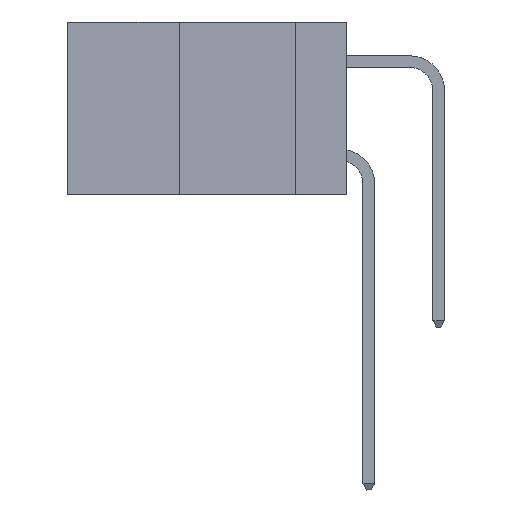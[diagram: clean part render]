
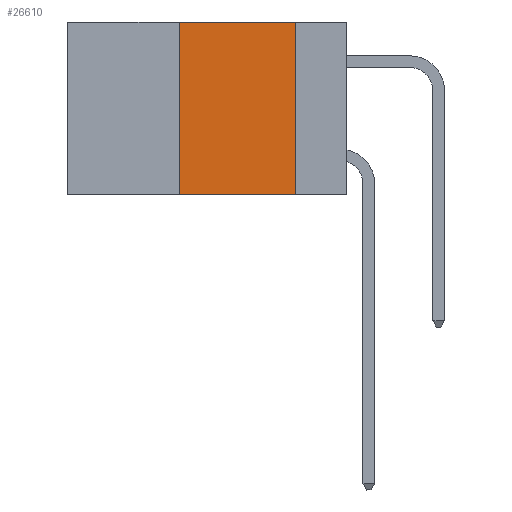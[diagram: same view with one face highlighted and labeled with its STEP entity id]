
A CAD part, left-side view. The second image highlights one B-rep face of the part: STEP entity #26610.
In plain terms, the highlighted planar face has unit normal (-1, 0, 0).
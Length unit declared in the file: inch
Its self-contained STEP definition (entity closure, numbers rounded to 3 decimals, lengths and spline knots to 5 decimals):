
#167 = CARTESIAN_POINT ( 'NONE',  ( 0., 0.6, 0. ) ) ;
#699 = ORIENTED_EDGE ( 'NONE', *, *, #12924, .T. ) ;
#1971 = LINE ( 'NONE', #6855, #19164 ) ;
#4062 = EDGE_CURVE ( 'NONE', #5437, #21570, #1971, .T. ) ;
#4903 = DIRECTION ( 'NONE',  ( 1., 0., 0. ) ) ;
#5437 = VERTEX_POINT ( 'NONE', #16604 ) ;
#6176 = LINE ( 'NONE', #27887, #16813 ) ;
#6855 = CARTESIAN_POINT ( 'NONE',  ( 0., 0.11, 0. ) ) ;
#7268 = ORIENTED_EDGE ( 'NONE', *, *, #13977, .F. ) ;
#8190 = FACE_OUTER_BOUND ( 'NONE', #28461, .T. ) ;
#9695 = LINE ( 'NONE', #13908, #23594 ) ;
#10172 = LINE ( 'NONE', #27730, #21498 ) ;
#11097 = ORIENTED_EDGE ( 'NONE', *, *, #4062, .F. ) ;
#12924 = EDGE_CURVE ( 'NONE', #26520, #21570, #6176, .T. ) ;
#13908 = CARTESIAN_POINT ( 'NONE',  ( 0., 0.6, 0. ) ) ;
#13977 = EDGE_CURVE ( 'NONE', #26520, #20164, #10172, .T. ) ;
#15837 = DIRECTION ( 'NONE',  ( 0., 0., 1. ) ) ;
#16360 = DIRECTION ( 'NONE',  ( 0., -1., 0. ) ) ;
#16604 = CARTESIAN_POINT ( 'NONE',  ( 0., 0.11, 0. ) ) ;
#16813 = VECTOR ( 'NONE', #18712, 39.37008 ) ;
#17507 = CARTESIAN_POINT ( 'NONE',  ( 0., 0.36, 0. ) ) ;
#18712 = DIRECTION ( 'NONE',  ( 0., -1., 0. ) ) ;
#19164 = VECTOR ( 'NONE', #27851, 39.37008 ) ;
#20164 = VERTEX_POINT ( 'NONE', #17507 ) ;
#21075 = CARTESIAN_POINT ( 'NONE',  ( 0., 0.36, -0.37 ) ) ;
#21394 = AXIS2_PLACEMENT_3D ( 'NONE', #167, #4903, #26064 ) ;
#21444 = EDGE_CURVE ( 'NONE', #20164, #5437, #9695, .T. ) ;
#21498 = VECTOR ( 'NONE', #15837, 39.37008 ) ;
#21570 = VERTEX_POINT ( 'NONE', #25738 ) ;
#23594 = VECTOR ( 'NONE', #16360, 39.37008 ) ;
#25738 = CARTESIAN_POINT ( 'NONE',  ( 0., 0.11, -0.37 ) ) ;
#26064 = DIRECTION ( 'NONE',  ( 0., 0., -1. ) ) ;
#26164 = PLANE ( 'NONE',  #21394 ) ;
#26520 = VERTEX_POINT ( 'NONE', #21075 ) ;
#26524 = ORIENTED_EDGE ( 'NONE', *, *, #21444, .F. ) ;
#26610 = ADVANCED_FACE ( 'NONE', ( #8190 ), #26164, .F. ) ;
#27730 = CARTESIAN_POINT ( 'NONE',  ( 0., 0.36, 0. ) ) ;
#27851 = DIRECTION ( 'NONE',  ( 0., 0., -1. ) ) ;
#27887 = CARTESIAN_POINT ( 'NONE',  ( 0., 0.6, -0.37 ) ) ;
#28461 = EDGE_LOOP ( 'NONE', ( #11097, #26524, #7268, #699 ) ) ;
